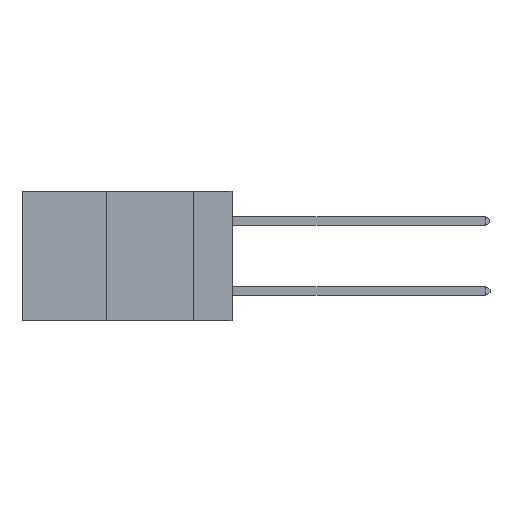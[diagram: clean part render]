
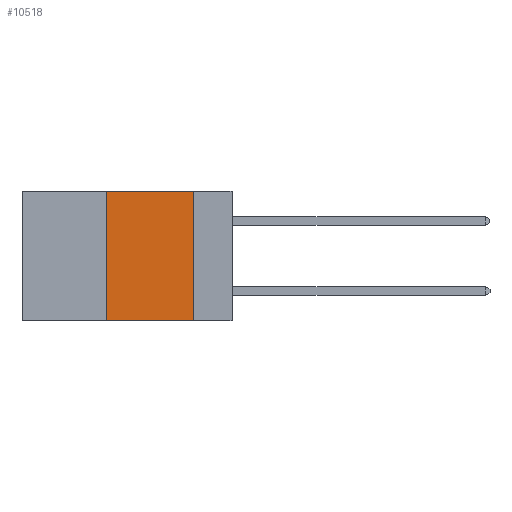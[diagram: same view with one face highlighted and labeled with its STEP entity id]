
A CAD part, left-side view. The second image highlights one B-rep face of the part: STEP entity #10518.
In plain terms, the highlighted planar face has unit normal (-1, 0, 0).
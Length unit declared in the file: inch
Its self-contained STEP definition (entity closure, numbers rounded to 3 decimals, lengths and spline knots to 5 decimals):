
#25 = CARTESIAN_POINT ( 'NONE',  ( 0., 0.36, 0. ) ) ;
#90 = VERTEX_POINT ( 'NONE', #2494 ) ;
#469 = VECTOR ( 'NONE', #842, 39.37008 ) ;
#472 = FACE_OUTER_BOUND ( 'NONE', #13467, .T. ) ;
#842 = DIRECTION ( 'NONE',  ( 0., 0., -1. ) ) ;
#1758 = DIRECTION ( 'NONE',  ( 0., 0., 1. ) ) ;
#2494 = CARTESIAN_POINT ( 'NONE',  ( 0., 0.36, -0.37 ) ) ;
#2668 = VERTEX_POINT ( 'NONE', #9700 ) ;
#3707 = VECTOR ( 'NONE', #4446, 39.37008 ) ;
#4446 = DIRECTION ( 'NONE',  ( 0., -1., 0. ) ) ;
#4711 = DIRECTION ( 'NONE',  ( 0., 0., -1. ) ) ;
#6573 = CARTESIAN_POINT ( 'NONE',  ( 0., 0.6, 0. ) ) ;
#6946 = VERTEX_POINT ( 'NONE', #9461 ) ;
#9461 = CARTESIAN_POINT ( 'NONE',  ( 0., 0.11, -0.37 ) ) ;
#9700 = CARTESIAN_POINT ( 'NONE',  ( 0., 0.36, 0. ) ) ;
#10518 = ADVANCED_FACE ( 'NONE', ( #472 ), #11540, .F. ) ;
#10923 = CARTESIAN_POINT ( 'NONE',  ( 0., 0.11, 0. ) ) ;
#11471 = CARTESIAN_POINT ( 'NONE',  ( 0., 0.6, 0. ) ) ;
#11519 = ORIENTED_EDGE ( 'NONE', *, *, #14904, .T. ) ;
#11540 = PLANE ( 'NONE',  #19999 ) ;
#12979 = VECTOR ( 'NONE', #1758, 39.37008 ) ;
#13467 = EDGE_LOOP ( 'NONE', ( #19209, #13896, #14561, #11519 ) ) ;
#13896 = ORIENTED_EDGE ( 'NONE', *, *, #18228, .F. ) ;
#14156 = LINE ( 'NONE', #21274, #469 ) ;
#14561 = ORIENTED_EDGE ( 'NONE', *, *, #20122, .F. ) ;
#14602 = VECTOR ( 'NONE', #15103, 39.37008 ) ;
#14904 = EDGE_CURVE ( 'NONE', #90, #6946, #17367, .T. ) ;
#14998 = DIRECTION ( 'NONE',  ( 1., 0., 0. ) ) ;
#15103 = DIRECTION ( 'NONE',  ( 0., -1., 0. ) ) ;
#15491 = EDGE_CURVE ( 'NONE', #16018, #6946, #14156, .T. ) ;
#16018 = VERTEX_POINT ( 'NONE', #10923 ) ;
#17367 = LINE ( 'NONE', #21510, #3707 ) ;
#18228 = EDGE_CURVE ( 'NONE', #2668, #16018, #19083, .T. ) ;
#18552 = LINE ( 'NONE', #25, #12979 ) ;
#19083 = LINE ( 'NONE', #6573, #14602 ) ;
#19209 = ORIENTED_EDGE ( 'NONE', *, *, #15491, .F. ) ;
#19999 = AXIS2_PLACEMENT_3D ( 'NONE', #11471, #14998, #4711 ) ;
#20122 = EDGE_CURVE ( 'NONE', #90, #2668, #18552, .T. ) ;
#21274 = CARTESIAN_POINT ( 'NONE',  ( 0., 0.11, 0. ) ) ;
#21510 = CARTESIAN_POINT ( 'NONE',  ( 0., 0.6, -0.37 ) ) ;
